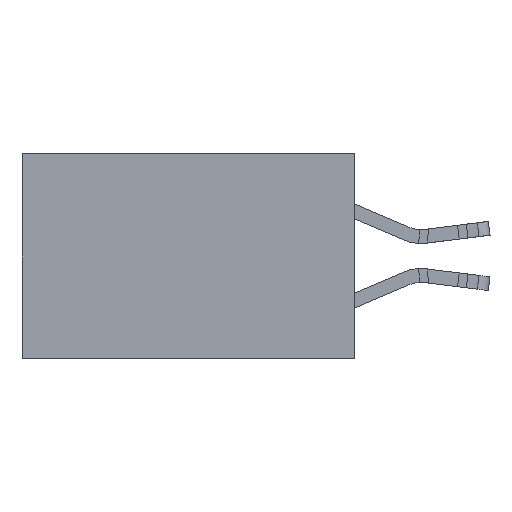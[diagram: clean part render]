
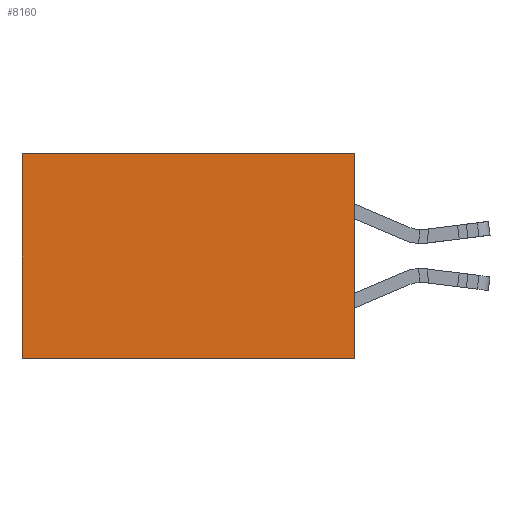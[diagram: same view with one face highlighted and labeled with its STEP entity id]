
A CAD part, left-side view. The second image highlights one B-rep face of the part: STEP entity #8160.
In plain terms, the highlighted planar face has unit normal (-1, 0, 0).
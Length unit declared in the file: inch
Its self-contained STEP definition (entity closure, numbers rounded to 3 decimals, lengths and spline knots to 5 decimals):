
#755 = CARTESIAN_POINT ( 'NONE',  ( 0.2615, 0., -0.37 ) ) ;
#1012 = CARTESIAN_POINT ( 'NONE',  ( 0.2615, 0.6, -0.37 ) ) ;
#1923 = VECTOR ( 'NONE', #6302, 39.37008 ) ;
#2429 = EDGE_CURVE ( 'NONE', #15617, #8914, #4810, .T. ) ;
#2595 = DIRECTION ( 'NONE',  ( 0., 0., -1. ) ) ;
#2601 = LINE ( 'NONE', #18826, #22267 ) ;
#2810 = CARTESIAN_POINT ( 'NONE',  ( 0.2615, 0., -0.37 ) ) ;
#4586 = LINE ( 'NONE', #25166, #22924 ) ;
#4810 = LINE ( 'NONE', #2810, #1923 ) ;
#5243 = VECTOR ( 'NONE', #2595, 39.37008 ) ;
#5983 = CARTESIAN_POINT ( 'NONE',  ( 0.2615, 0.6, -0.37 ) ) ;
#6302 = DIRECTION ( 'NONE',  ( 0., 1., 0. ) ) ;
#6396 = CARTESIAN_POINT ( 'NONE',  ( 0.2615, 0.6, 0. ) ) ;
#7071 = DIRECTION ( 'NONE',  ( 0., 1., 0. ) ) ;
#8160 = ADVANCED_FACE ( 'NONE', ( #20930 ), #14488, .F. ) ;
#8914 = VERTEX_POINT ( 'NONE', #5983 ) ;
#9569 = CARTESIAN_POINT ( 'NONE',  ( 0.2615, 0., -0.37 ) ) ;
#9937 = ORIENTED_EDGE ( 'NONE', *, *, #18126, .T. ) ;
#10639 = DIRECTION ( 'NONE',  ( 0., 0., -1. ) ) ;
#11285 = EDGE_LOOP ( 'NONE', ( #9937, #19185, #17377, #24849 ) ) ;
#11610 = CARTESIAN_POINT ( 'NONE',  ( 0.2615, 0., 0. ) ) ;
#13278 = LINE ( 'NONE', #1012, #5243 ) ;
#14488 = PLANE ( 'NONE',  #16803 ) ;
#15617 = VERTEX_POINT ( 'NONE', #9569 ) ;
#16803 = AXIS2_PLACEMENT_3D ( 'NONE', #755, #22552, #24918 ) ;
#16841 = EDGE_CURVE ( 'NONE', #22551, #25120, #4586, .T. ) ;
#17377 = ORIENTED_EDGE ( 'NONE', *, *, #23216, .F. ) ;
#18126 = EDGE_CURVE ( 'NONE', #25120, #8914, #13278, .T. ) ;
#18826 = CARTESIAN_POINT ( 'NONE',  ( 0.2615, 0., -0.37 ) ) ;
#19185 = ORIENTED_EDGE ( 'NONE', *, *, #2429, .F. ) ;
#20930 = FACE_OUTER_BOUND ( 'NONE', #11285, .T. ) ;
#22267 = VECTOR ( 'NONE', #10639, 39.37008 ) ;
#22551 = VERTEX_POINT ( 'NONE', #11610 ) ;
#22552 = DIRECTION ( 'NONE',  ( 1., 0., 0. ) ) ;
#22924 = VECTOR ( 'NONE', #7071, 39.37008 ) ;
#23216 = EDGE_CURVE ( 'NONE', #22551, #15617, #2601, .T. ) ;
#24849 = ORIENTED_EDGE ( 'NONE', *, *, #16841, .T. ) ;
#24918 = DIRECTION ( 'NONE',  ( 0., 0., -1. ) ) ;
#25120 = VERTEX_POINT ( 'NONE', #6396 ) ;
#25166 = CARTESIAN_POINT ( 'NONE',  ( 0.2615, 0., 0. ) ) ;
